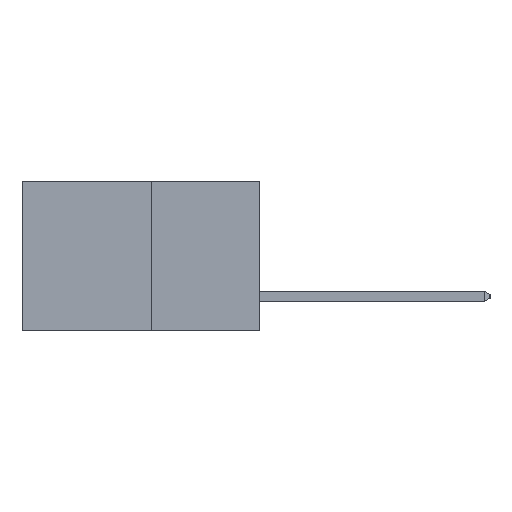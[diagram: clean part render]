
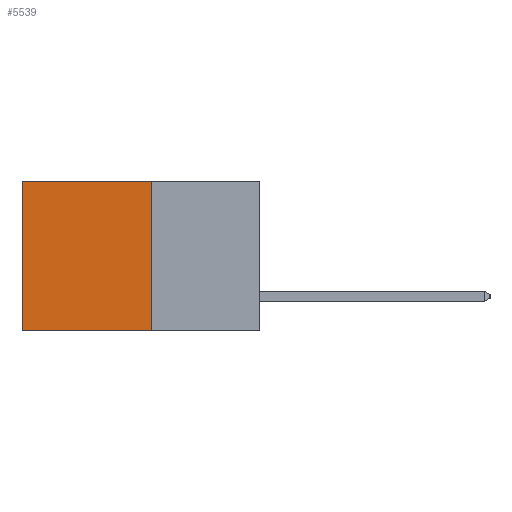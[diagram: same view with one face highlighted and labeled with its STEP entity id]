
A CAD part, left-side view. The second image highlights one B-rep face of the part: STEP entity #5539.
In plain terms, the highlighted planar face has unit normal (-1, 0, 0).
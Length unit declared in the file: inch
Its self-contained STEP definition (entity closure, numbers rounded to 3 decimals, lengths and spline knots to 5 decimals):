
#36 = DIRECTION ( 'NONE',  ( 0., 1., 0. ) ) ;
#122 = DIRECTION ( 'NONE',  ( 1., 0., 0. ) ) ;
#155 = CARTESIAN_POINT ( 'NONE',  ( 0.277, 0.27, -0.37 ) ) ;
#249 = ORIENTED_EDGE ( 'NONE', *, *, #6655, .F. ) ;
#389 = ORIENTED_EDGE ( 'NONE', *, *, #3268, .F. ) ;
#552 = CARTESIAN_POINT ( 'NONE',  ( 0.277, 0.27, -0.37 ) ) ;
#825 = ORIENTED_EDGE ( 'NONE', *, *, #5421, .T. ) ;
#1066 = FACE_OUTER_BOUND ( 'NONE', #6563, .T. ) ;
#1100 = VERTEX_POINT ( 'NONE', #6632 ) ;
#1973 = DIRECTION ( 'NONE',  ( 0., 0., -1. ) ) ;
#2097 = EDGE_CURVE ( 'NONE', #7784, #1100, #3009, .T. ) ;
#2616 = VERTEX_POINT ( 'NONE', #2783 ) ;
#2636 = ORIENTED_EDGE ( 'NONE', *, *, #2097, .T. ) ;
#2725 = VERTEX_POINT ( 'NONE', #5343 ) ;
#2783 = CARTESIAN_POINT ( 'NONE',  ( 0.277, 0.59, -0.37 ) ) ;
#2795 = VECTOR ( 'NONE', #3089, 39.37008 ) ;
#3009 = LINE ( 'NONE', #3141, #2795 ) ;
#3089 = DIRECTION ( 'NONE',  ( 0., 1., 0. ) ) ;
#3141 = CARTESIAN_POINT ( 'NONE',  ( 0.277, 0.27, 0. ) ) ;
#3268 = EDGE_CURVE ( 'NONE', #7784, #2725, #5907, .T. ) ;
#3635 = LINE ( 'NONE', #6120, #6795 ) ;
#3675 = PLANE ( 'NONE',  #5420 ) ;
#3857 = DIRECTION ( 'NONE',  ( 0., 0., -1. ) ) ;
#4007 = VECTOR ( 'NONE', #6440, 39.37008 ) ;
#4032 = VECTOR ( 'NONE', #36, 39.37008 ) ;
#4213 = CARTESIAN_POINT ( 'NONE',  ( 0.277, 0.27, -0.37 ) ) ;
#5343 = CARTESIAN_POINT ( 'NONE',  ( 0.277, 0.27, -0.37 ) ) ;
#5420 = AXIS2_PLACEMENT_3D ( 'NONE', #155, #122, #3857 ) ;
#5421 = EDGE_CURVE ( 'NONE', #1100, #2616, #3635, .T. ) ;
#5539 = ADVANCED_FACE ( 'NONE', ( #1066 ), #3675, .F. ) ;
#5907 = LINE ( 'NONE', #4213, #4007 ) ;
#5922 = LINE ( 'NONE', #552, #4032 ) ;
#6120 = CARTESIAN_POINT ( 'NONE',  ( 0.277, 0.59, -0.37 ) ) ;
#6440 = DIRECTION ( 'NONE',  ( 0., 0., -1. ) ) ;
#6538 = CARTESIAN_POINT ( 'NONE',  ( 0.277, 0.27, 0. ) ) ;
#6563 = EDGE_LOOP ( 'NONE', ( #825, #249, #389, #2636 ) ) ;
#6632 = CARTESIAN_POINT ( 'NONE',  ( 0.277, 0.59, 0. ) ) ;
#6655 = EDGE_CURVE ( 'NONE', #2725, #2616, #5922, .T. ) ;
#6795 = VECTOR ( 'NONE', #1973, 39.37008 ) ;
#7784 = VERTEX_POINT ( 'NONE', #6538 ) ;
